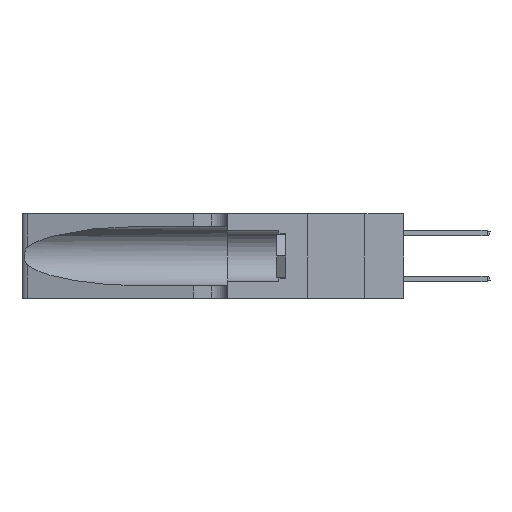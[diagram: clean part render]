
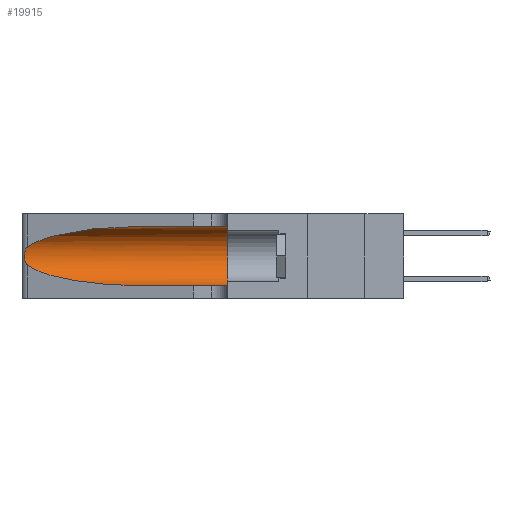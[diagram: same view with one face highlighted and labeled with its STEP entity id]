
A CAD part, left-side view. The second image highlights one B-rep face of the part: STEP entity #19915.
In plain terms, the highlighted cylindrical face has radius 3.308 mm (diameter 6.617 mm), a partial arc.
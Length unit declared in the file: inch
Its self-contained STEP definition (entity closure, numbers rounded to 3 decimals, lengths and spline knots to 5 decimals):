
#523 = CARTESIAN_POINT ( 'NONE',  ( 0.26075, 1.23896, 0.178 ) ) ;
#1730 = DIRECTION ( 'NONE',  ( 0., 0., 1. ) ) ;
#1784 = CARTESIAN_POINT ( 'NONE',  ( 0.1305, 1.61858, 0.31525 ) ) ;
#2782 = DIRECTION ( 'NONE',  ( 0., -1., 0. ) ) ;
#3777 = CARTESIAN_POINT ( 'NONE',  ( 0.2373, 1.15595, 0.08982 ) ) ;
#3915 = CARTESIAN_POINT ( 'NONE',  ( 0.25856, 1.23593, 0.16098 ) ) ;
#5220 =( BOUNDED_CURVE ( )  B_SPLINE_CURVE ( 3, ( #10627, #3777, #20678, #34217 ),
 .UNSPECIFIED., .F., .F. ) 
 B_SPLINE_CURVE_WITH_KNOTS ( ( 4, 4 ),
 ( 3.44316, 4.71239 ),
 .UNSPECIFIED. ) 
 CURVE ( )  GEOMETRIC_REPRESENTATION_ITEM ( )  RATIONAL_B_SPLINE_CURVE ( ( 1., 0.87, 0.87, 1. ) ) 
 REPRESENTATION_ITEM ( '' )  );
#6368 = LINE ( 'NONE', #1784, #31219 ) ;
#6975 = CIRCLE ( 'NONE', #27263, 0.13025 ) ;
#7205 = CARTESIAN_POINT ( 'NONE',  ( 0.25555, 1.22994, 0.2215 ) ) ;
#7352 = CARTESIAN_POINT ( 'NONE',  ( 0.25639, 1.23186, 0.15144 ) ) ;
#9459 = CARTESIAN_POINT ( 'NONE',  ( 0.1305, 1.61858, 0.05475 ) ) ;
#10627 = CARTESIAN_POINT ( 'NONE',  ( 0.25487, 1.22718, 0.14631 ) ) ;
#10766 = CARTESIAN_POINT ( 'NONE',  ( 0.25487, 1.22718, 0.14631 ) ) ;
#11937 = CARTESIAN_POINT ( 'NONE',  ( 0.1305, 0.35, 0.05475 ) ) ;
#12681 = EDGE_CURVE ( 'NONE', #32547, #28700, #20992, .T. ) ;
#13871 = ORIENTED_EDGE ( 'NONE', *, *, #12681, .T. ) ;
#14005 = CARTESIAN_POINT ( 'NONE',  ( 0.25639, 1.23184, 0.21858 ) ) ;
#14427 = EDGE_LOOP ( 'NONE', ( #13871, #19212, #40246, #23426, #39832, #30433 ) ) ;
#15421 = DIRECTION ( 'NONE',  ( 0., 0., -1. ) ) ;
#16390 = CARTESIAN_POINT ( 'NONE',  ( 0.18966, 0.96281, 0.31525 ) ) ;
#17415 = CARTESIAN_POINT ( 'NONE',  ( 0.25854, 1.2359, 0.20912 ) ) ;
#19212 = ORIENTED_EDGE ( 'NONE', *, *, #36601, .T. ) ;
#19823 = CARTESIAN_POINT ( 'NONE',  ( 0.2373, 1.15595, 0.28018 ) ) ;
#19915 = ADVANCED_FACE ( 'NONE', ( #40680 ), #30726, .F. ) ;
#20653 = EDGE_CURVE ( 'NONE', #42704, #38773, #35861, .T. ) ;
#20678 = CARTESIAN_POINT ( 'NONE',  ( 0.18966, 0.96281, 0.05475 ) ) ;
#20823 = CARTESIAN_POINT ( 'NONE',  ( 0.26075, 1.23896, 0.19203 ) ) ;
#20851 = EDGE_CURVE ( 'NONE', #39749, #42704, #5220, .T. ) ;
#20992 =( BOUNDED_CURVE ( )  B_SPLINE_CURVE ( 3, ( #39941, #16390, #19823, #43337 ),
 .UNSPECIFIED., .F., .T. ) 
 B_SPLINE_CURVE_WITH_KNOTS ( ( 4, 4 ),
 ( 1.5708, 2.84003 ),
 .UNSPECIFIED. ) 
 CURVE ( )  GEOMETRIC_REPRESENTATION_ITEM ( )  RATIONAL_B_SPLINE_CURVE ( ( 1., 0.87, 0.87, 1. ) ) 
 REPRESENTATION_ITEM ( '' )  );
#21304 = VERTEX_POINT ( 'NONE', #35152 ) ;
#21852 = CARTESIAN_POINT ( 'NONE',  ( 0.1305, 0.72297, 0.31525 ) ) ;
#22003 = DIRECTION ( 'NONE',  ( 0., 1., 0. ) ) ;
#23426 = ORIENTED_EDGE ( 'NONE', *, *, #20653, .T. ) ;
#24206 = CARTESIAN_POINT ( 'NONE',  ( 0.26017, 1.23833, 0.17102 ) ) ;
#25823 = CARTESIAN_POINT ( 'NONE',  ( 0.1305, 0.72297, 0.05475 ) ) ;
#26454 = CARTESIAN_POINT ( 'NONE',  ( 0.25487, 1.22718, 0.14631 ) ) ;
#26945 = VECTOR ( 'NONE', #2782, 39.37008 ) ;
#27263 = AXIS2_PLACEMENT_3D ( 'NONE', #42141, #22003, #1730 ) ;
#27590 = CARTESIAN_POINT ( 'NONE',  ( 0.25789, 1.23486, 0.15765 ) ) ;
#28700 = VERTEX_POINT ( 'NONE', #39724 ) ;
#28874 = CARTESIAN_POINT ( 'NONE',  ( 0.1305, 1.61858, 0.185 ) ) ;
#29254 = EDGE_CURVE ( 'NONE', #32547, #21304, #6368, .T. ) ;
#30180 = AXIS2_PLACEMENT_3D ( 'NONE', #28874, #35588, #15421 ) ;
#30433 = ORIENTED_EDGE ( 'NONE', *, *, #29254, .F. ) ;
#30726 = CYLINDRICAL_SURFACE ( 'NONE', #30180, 0.13025 ) ;
#30861 = CARTESIAN_POINT ( 'NONE',  ( 0.25487, 1.22718, 0.22369 ) ) ;
#31006 = CARTESIAN_POINT ( 'NONE',  ( 0.25555, 1.22993, 0.14849 ) ) ;
#31219 = VECTOR ( 'NONE', #32366, 39.37008 ) ;
#32366 = DIRECTION ( 'NONE',  ( 0., -1., 0. ) ) ;
#32547 = VERTEX_POINT ( 'NONE', #21852 ) ;
#34217 = CARTESIAN_POINT ( 'NONE',  ( 0.1305, 0.72297, 0.05475 ) ) ;
#35152 = CARTESIAN_POINT ( 'NONE',  ( 0.1305, 0.35, 0.31525 ) ) ;
#35588 = DIRECTION ( 'NONE',  ( 0., -1., 0. ) ) ;
#35861 = LINE ( 'NONE', #9459, #26945 ) ;
#36601 = EDGE_CURVE ( 'NONE', #28700, #39749, #37940, .T. ) ;
#37559 = CARTESIAN_POINT ( 'NONE',  ( 0.25787, 1.23484, 0.2124 ) ) ;
#37940 = B_SPLINE_CURVE_WITH_KNOTS ( 'NONE', 3,
 ( #30861, #7205, #14005, #37559, #17415, #40961, #20823, #523, #24206, #3915, #27590, #7352, #31006, #10766 ),
 .UNSPECIFIED., .F., .F.,
 ( 4, 2, 2, 2, 2, 2, 4 ),
 ( 0., 0.00027, 0.00053, 0.00107, 0.0016, 0.00187, 0.00214 ),
 .UNSPECIFIED. ) ;
#38773 = VERTEX_POINT ( 'NONE', #11937 ) ;
#39724 = CARTESIAN_POINT ( 'NONE',  ( 0.25487, 1.22718, 0.22369 ) ) ;
#39749 = VERTEX_POINT ( 'NONE', #26454 ) ;
#39832 = ORIENTED_EDGE ( 'NONE', *, *, #40196, .F. ) ;
#39941 = CARTESIAN_POINT ( 'NONE',  ( 0.1305, 0.72297, 0.31525 ) ) ;
#40196 = EDGE_CURVE ( 'NONE', #21304, #38773, #6975, .T. ) ;
#40246 = ORIENTED_EDGE ( 'NONE', *, *, #20851, .T. ) ;
#40680 = FACE_OUTER_BOUND ( 'NONE', #14427, .T. ) ;
#40961 = CARTESIAN_POINT ( 'NONE',  ( 0.26018, 1.23835, 0.19895 ) ) ;
#42141 = CARTESIAN_POINT ( 'NONE',  ( 0.1305, 0.35, 0.185 ) ) ;
#42704 = VERTEX_POINT ( 'NONE', #25823 ) ;
#43337 = CARTESIAN_POINT ( 'NONE',  ( 0.25487, 1.22718, 0.22369 ) ) ;
